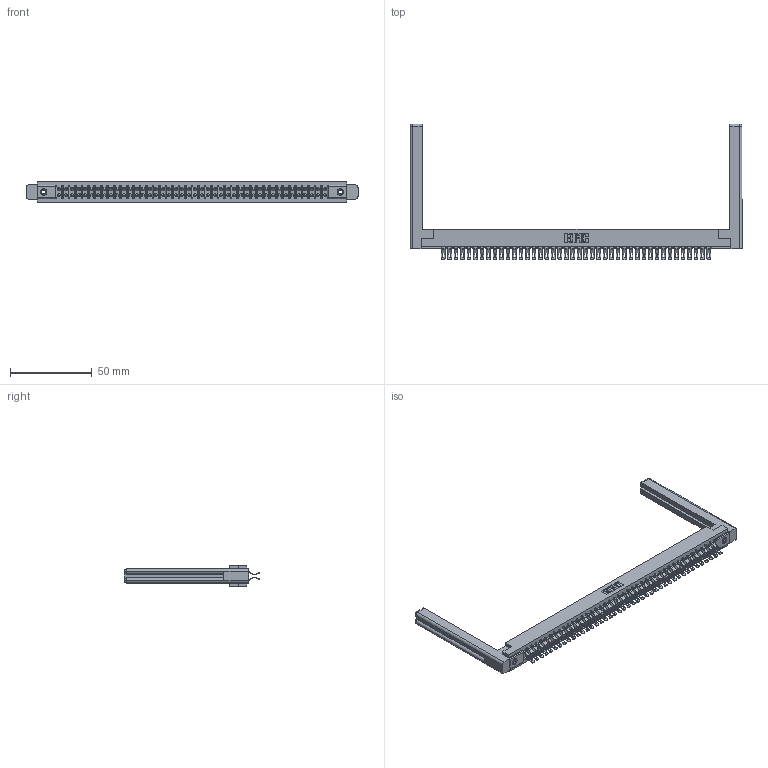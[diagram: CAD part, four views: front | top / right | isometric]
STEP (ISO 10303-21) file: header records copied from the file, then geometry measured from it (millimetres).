
FILE_DESCRIPTION (( 'STEP AP203' ), '1' );
FILE_NAME ('357-084-555-258.STEP', '2019-09-19T18:09:26', ( '' ), ( '' ), 'SwSTEP 2.0', 'SolidWorks 2016', '' );
FILE_SCHEMA (( 'CONFIG_CONTROL_DESIGN' ));
Length unit declared in the file: inch
Products named in the file (5): 307-290-001_555; 307 Part_.156 Dia Mounting Holes; 357-084-555-258; 307-220-058; 345-250-001_345-250-001-102
Assembly tree (89 placements, depth 2):
  357-084-555-258
    307 Part_.156 Dia Mounting Holes
    307-290-001_555  x84
    307-220-058  x2
    345-250-001_345-250-001-102  x2
Bounding box: 203.05 x 83.06 x 12.7 mm (x, y, z)
Volume: 28971.4 mm3; surface area: 33007.5 mm2
Topology: 89 solids, 89 shells, 5427 faces, 15881 edges, 10346 vertices
Faces by surface type: plane 3010, cylinder 2307, sphere 86, torus 12, cone 12
Entity records: 40520 total; most frequent: CARTESIAN_POINT 6653, ORIENTED_EDGE 6538, DIRECTION 6481, EDGE_CURVE 3269, VECTOR 2493, LINE 2493, VERTEX_POINT 2112, AXIS2_PLACEMENT_3D 1994
